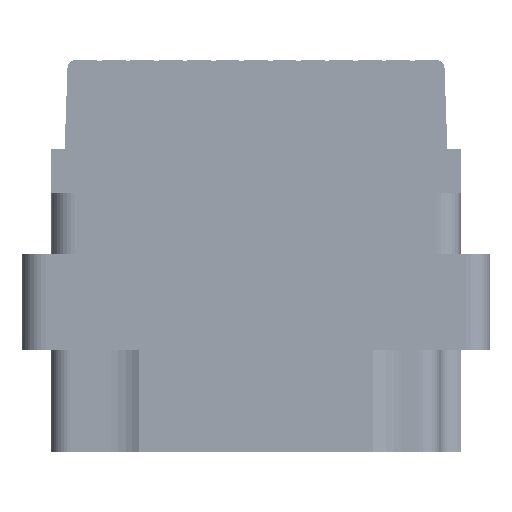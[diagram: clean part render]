
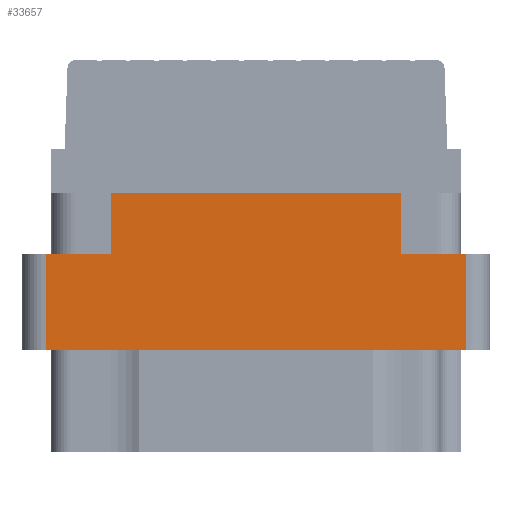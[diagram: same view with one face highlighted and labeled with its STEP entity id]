
A CAD part, left-side view. The second image highlights one B-rep face of the part: STEP entity #33657.
In plain terms, the highlighted planar face has unit normal (-1, 0, 0).
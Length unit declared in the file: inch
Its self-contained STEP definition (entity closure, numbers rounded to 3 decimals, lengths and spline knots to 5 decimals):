
#601 = AXIS2_PLACEMENT_3D ( 'NONE', #4245, #33131, #26395 ) ;
#2391 = EDGE_CURVE ( 'NONE', #12111, #68448, #32947, .T. ) ;
#3440 = CARTESIAN_POINT ( 'NONE',  ( -1.359, -0.555, -0.277 ) ) ;
#4245 = CARTESIAN_POINT ( 'NONE',  ( -1.359, -0.617, -0.798 ) ) ;
#5166 = VERTEX_POINT ( 'NONE', #56750 ) ;
#8852 = CARTESIAN_POINT ( 'NONE',  ( -1.359, -0.3825, -0.117 ) ) ;
#9333 = DIRECTION ( 'NONE',  ( 0., 0., 1. ) ) ;
#11123 = LINE ( 'NONE', #16760, #25039 ) ;
#12111 = VERTEX_POINT ( 'NONE', #42488 ) ;
#12197 = LINE ( 'NONE', #40345, #70356 ) ;
#16108 = DIRECTION ( 'NONE',  ( 0., -1., 0. ) ) ;
#16201 = DIRECTION ( 'NONE',  ( 0., 1., 0. ) ) ;
#16760 = CARTESIAN_POINT ( 'NONE',  ( -1.359, 0.617, -0.117 ) ) ;
#18491 = CARTESIAN_POINT ( 'NONE',  ( -1.359, 0.555, -0.529 ) ) ;
#19618 = EDGE_CURVE ( 'NONE', #47737, #58579, #49940, .T. ) ;
#19901 = VECTOR ( 'NONE', #28081, 39.37008 ) ;
#20005 = ORIENTED_EDGE ( 'NONE', *, *, #2391, .F. ) ;
#20233 = LINE ( 'NONE', #42755, #68813 ) ;
#21867 = PLANE ( 'NONE',  #601 ) ;
#22191 = CARTESIAN_POINT ( 'NONE',  ( -1.359, 0., -0.529 ) ) ;
#25039 = VECTOR ( 'NONE', #68910, 39.37008 ) ;
#25266 = VECTOR ( 'NONE', #16201, 39.37008 ) ;
#26395 = DIRECTION ( 'NONE',  ( 0., 0., 1. ) ) ;
#28081 = DIRECTION ( 'NONE',  ( 0., 0., 1. ) ) ;
#28384 = ORIENTED_EDGE ( 'NONE', *, *, #19618, .T. ) ;
#28788 = ORIENTED_EDGE ( 'NONE', *, *, #52387, .F. ) ;
#28802 = EDGE_LOOP ( 'NONE', ( #63151, #28384, #44956, #54372, #72580, #66978, #28788, #20005 ) ) ;
#29091 = DIRECTION ( 'NONE',  ( 0., -1., 0. ) ) ;
#31835 = VERTEX_POINT ( 'NONE', #8852 ) ;
#32298 = CARTESIAN_POINT ( 'NONE',  ( -1.359, 0.555, -0.798 ) ) ;
#32947 = LINE ( 'NONE', #56203, #41177 ) ;
#33131 = DIRECTION ( 'NONE',  ( -1., 0., 0. ) ) ;
#33657 = ADVANCED_FACE ( 'NONE', ( #43301 ), #21867, .T. ) ;
#35107 = VECTOR ( 'NONE', #16108, 39.37008 ) ;
#35500 = CARTESIAN_POINT ( 'NONE',  ( -1.359, 0.555, -0.277 ) ) ;
#40068 = CARTESIAN_POINT ( 'NONE',  ( -1.359, -0.3825, -0.277 ) ) ;
#40345 = CARTESIAN_POINT ( 'NONE',  ( -1.359, 0., -0.277 ) ) ;
#41177 = VECTOR ( 'NONE', #43500, 39.37008 ) ;
#42488 = CARTESIAN_POINT ( 'NONE',  ( -1.359, 0.3825, -0.277 ) ) ;
#42755 = CARTESIAN_POINT ( 'NONE',  ( -1.359, -0.555, -0.798 ) ) ;
#43210 = VERTEX_POINT ( 'NONE', #64323 ) ;
#43301 = FACE_OUTER_BOUND ( 'NONE', #28802, .T. ) ;
#43500 = DIRECTION ( 'NONE',  ( 0., 0., 1. ) ) ;
#44364 = LINE ( 'NONE', #22191, #25266 ) ;
#44956 = ORIENTED_EDGE ( 'NONE', *, *, #56449, .F. ) ;
#45562 = EDGE_CURVE ( 'NONE', #5166, #62850, #20233, .T. ) ;
#47737 = VERTEX_POINT ( 'NONE', #35500 ) ;
#48792 = LINE ( 'NONE', #58557, #35107 ) ;
#49940 = LINE ( 'NONE', #32298, #65689 ) ;
#52387 = EDGE_CURVE ( 'NONE', #68448, #31835, #11123, .T. ) ;
#54372 = ORIENTED_EDGE ( 'NONE', *, *, #45562, .T. ) ;
#56203 = CARTESIAN_POINT ( 'NONE',  ( -1.359, 0.3825, -0.277 ) ) ;
#56449 = EDGE_CURVE ( 'NONE', #5166, #58579, #44364, .T. ) ;
#56750 = CARTESIAN_POINT ( 'NONE',  ( -1.359, -0.555, -0.529 ) ) ;
#58557 = CARTESIAN_POINT ( 'NONE',  ( -1.359, 0., -0.277 ) ) ;
#58579 = VERTEX_POINT ( 'NONE', #18491 ) ;
#60473 = EDGE_CURVE ( 'NONE', #47737, #12111, #48792, .T. ) ;
#61925 = DIRECTION ( 'NONE',  ( 0., 0., -1. ) ) ;
#62850 = VERTEX_POINT ( 'NONE', #3440 ) ;
#63151 = ORIENTED_EDGE ( 'NONE', *, *, #60473, .F. ) ;
#64323 = CARTESIAN_POINT ( 'NONE',  ( -1.359, -0.3825, -0.277 ) ) ;
#65689 = VECTOR ( 'NONE', #61925, 39.37008 ) ;
#66978 = ORIENTED_EDGE ( 'NONE', *, *, #68951, .T. ) ;
#67861 = LINE ( 'NONE', #40068, #19901 ) ;
#68448 = VERTEX_POINT ( 'NONE', #69931 ) ;
#68813 = VECTOR ( 'NONE', #9333, 39.37008 ) ;
#68910 = DIRECTION ( 'NONE',  ( 0., -1., 0. ) ) ;
#68951 = EDGE_CURVE ( 'NONE', #43210, #31835, #67861, .T. ) ;
#69931 = CARTESIAN_POINT ( 'NONE',  ( -1.359, 0.3825, -0.117 ) ) ;
#70326 = EDGE_CURVE ( 'NONE', #43210, #62850, #12197, .T. ) ;
#70356 = VECTOR ( 'NONE', #29091, 39.37008 ) ;
#72580 = ORIENTED_EDGE ( 'NONE', *, *, #70326, .F. ) ;
